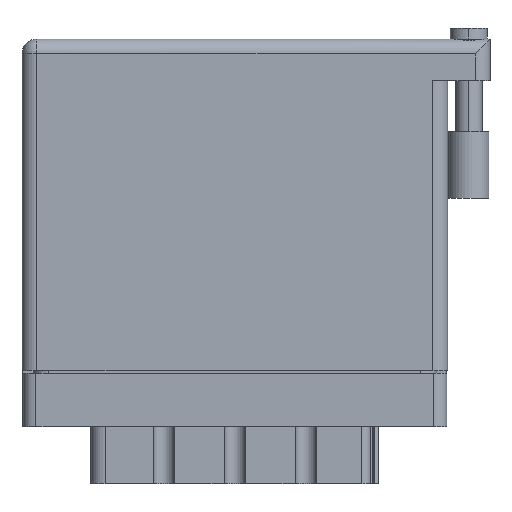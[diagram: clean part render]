
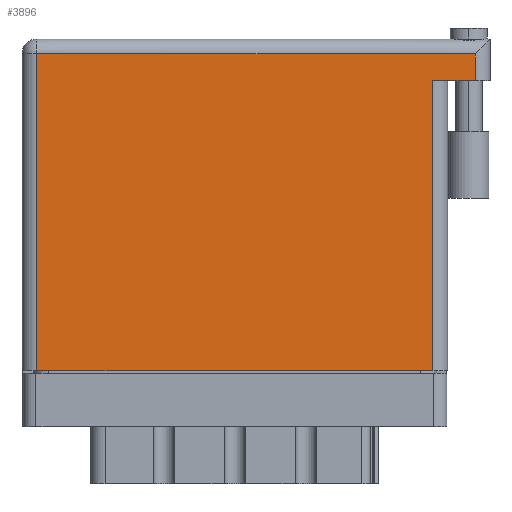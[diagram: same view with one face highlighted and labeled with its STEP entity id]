
A CAD part, front view. The second image highlights one B-rep face of the part: STEP entity #3896.
In plain terms, the highlighted face is planar.
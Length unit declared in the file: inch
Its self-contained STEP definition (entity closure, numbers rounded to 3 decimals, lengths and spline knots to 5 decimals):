
#751 = DIRECTION ( 'NONE',  ( 1., 0., 0. ) ) ;
#1388 = CARTESIAN_POINT ( 'NONE',  ( 1.938, 1.369, 0. ) ) ;
#1474 = VERTEX_POINT ( 'NONE', #16641 ) ;
#1649 = EDGE_LOOP ( 'NONE', ( #19685, #32098, #16978, #10592, #12350, #17830 ) ) ;
#2815 = VERTEX_POINT ( 'NONE', #4063 ) ;
#3518 = VERTEX_POINT ( 'NONE', #4535 ) ;
#3872 = VECTOR ( 'NONE', #27661, 39.37008 ) ;
#3896 = ADVANCED_FACE ( 'NONE', ( #25284 ), #21742, .F. ) ;
#4063 = CARTESIAN_POINT ( 'NONE',  ( 2.138, 1.496, 0. ) ) ;
#4393 = DIRECTION ( 'NONE',  ( 0., 1., 0. ) ) ;
#4535 = CARTESIAN_POINT ( 'NONE',  ( 0.07, 0., 0. ) ) ;
#4790 = DIRECTION ( 'NONE',  ( 0., 1., 0. ) ) ;
#6513 = LINE ( 'NONE', #10009, #24042 ) ;
#6516 = DIRECTION ( 'NONE',  ( 0., 0., -1. ) ) ;
#7253 = CARTESIAN_POINT ( 'NONE',  ( 2.208, 1.369, 0. ) ) ;
#7622 = CARTESIAN_POINT ( 'NONE',  ( 1.938, 0., 0. ) ) ;
#8142 = CARTESIAN_POINT ( 'NONE',  ( 0.07, 1.496, 0. ) ) ;
#9212 = LINE ( 'NONE', #23543, #27558 ) ;
#9943 = DIRECTION ( 'NONE',  ( 0., -1., 0. ) ) ;
#10009 = CARTESIAN_POINT ( 'NONE',  ( 2.138, 1.566, 0. ) ) ;
#10291 = VECTOR ( 'NONE', #4393, 39.37008 ) ;
#10592 = ORIENTED_EDGE ( 'NONE', *, *, #25885, .T. ) ;
#10639 = VERTEX_POINT ( 'NONE', #1388 ) ;
#12313 = EDGE_CURVE ( 'NONE', #15315, #10639, #26670, .T. ) ;
#12350 = ORIENTED_EDGE ( 'NONE', *, *, #17899, .T. ) ;
#13235 = VECTOR ( 'NONE', #9943, 39.37008 ) ;
#14155 = CARTESIAN_POINT ( 'NONE',  ( 0., 1.566, 0. ) ) ;
#15055 = AXIS2_PLACEMENT_3D ( 'NONE', #14155, #6516, #18944 ) ;
#15315 = VERTEX_POINT ( 'NONE', #7622 ) ;
#15652 = VECTOR ( 'NONE', #17346, 39.37008 ) ;
#16641 = CARTESIAN_POINT ( 'NONE',  ( 2.138, 1.369, 0. ) ) ;
#16978 = ORIENTED_EDGE ( 'NONE', *, *, #25849, .F. ) ;
#17346 = DIRECTION ( 'NONE',  ( -1., 0., 0. ) ) ;
#17830 = ORIENTED_EDGE ( 'NONE', *, *, #20189, .T. ) ;
#17899 = EDGE_CURVE ( 'NONE', #2815, #32630, #28184, .T. ) ;
#18944 = DIRECTION ( 'NONE',  ( -1., 0., 0. ) ) ;
#19685 = ORIENTED_EDGE ( 'NONE', *, *, #30262, .T. ) ;
#19994 = LINE ( 'NONE', #29902, #13235 ) ;
#20189 = EDGE_CURVE ( 'NONE', #32630, #3518, #19994, .T. ) ;
#21635 = LINE ( 'NONE', #7253, #15652 ) ;
#21742 = PLANE ( 'NONE',  #15055 ) ;
#23543 = CARTESIAN_POINT ( 'NONE',  ( 0., 0., 0. ) ) ;
#24042 = VECTOR ( 'NONE', #4790, 39.37008 ) ;
#24866 = CARTESIAN_POINT ( 'NONE',  ( 1.938, 1.369, 0. ) ) ;
#25284 = FACE_OUTER_BOUND ( 'NONE', #1649, .T. ) ;
#25849 = EDGE_CURVE ( 'NONE', #1474, #10639, #21635, .T. ) ;
#25885 = EDGE_CURVE ( 'NONE', #1474, #2815, #6513, .T. ) ;
#26670 = LINE ( 'NONE', #24866, #10291 ) ;
#27558 = VECTOR ( 'NONE', #751, 39.37008 ) ;
#27661 = DIRECTION ( 'NONE',  ( -1., 0., 0. ) ) ;
#28184 = LINE ( 'NONE', #29897, #3872 ) ;
#29897 = CARTESIAN_POINT ( 'NONE',  ( 0., 1.496, 0. ) ) ;
#29902 = CARTESIAN_POINT ( 'NONE',  ( 0.07, 0., 0. ) ) ;
#30262 = EDGE_CURVE ( 'NONE', #3518, #15315, #9212, .T. ) ;
#32098 = ORIENTED_EDGE ( 'NONE', *, *, #12313, .T. ) ;
#32630 = VERTEX_POINT ( 'NONE', #8142 ) ;
